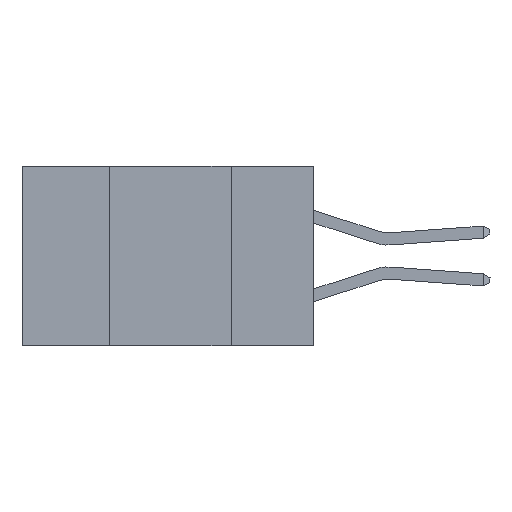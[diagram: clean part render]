
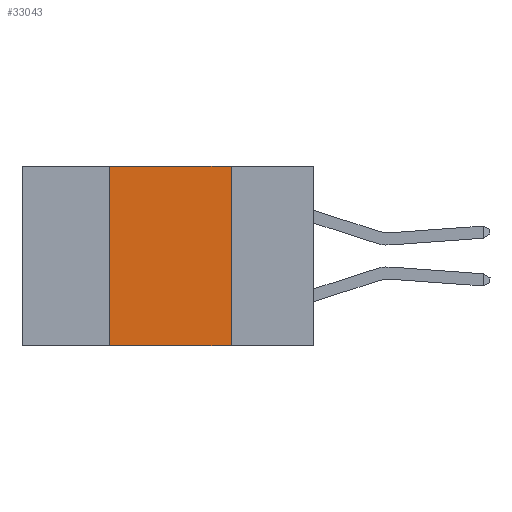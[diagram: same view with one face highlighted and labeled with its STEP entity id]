
A CAD part, left-side view. The second image highlights one B-rep face of the part: STEP entity #33043.
In plain terms, the highlighted planar face has unit normal (-1, 0, 0).
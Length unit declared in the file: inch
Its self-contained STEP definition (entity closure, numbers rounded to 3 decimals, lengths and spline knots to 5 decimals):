
#213 = PLANE ( 'NONE',  #12985 ) ;
#1413 = EDGE_CURVE ( 'NONE', #13924, #30875, #5237, .T. ) ;
#2487 = VERTEX_POINT ( 'NONE', #26704 ) ;
#2660 = CARTESIAN_POINT ( 'NONE',  ( 0., 0.17, -0.37 ) ) ;
#3637 = DIRECTION ( 'NONE',  ( 0., 0., -1. ) ) ;
#5237 = LINE ( 'NONE', #24204, #24035 ) ;
#6489 = DIRECTION ( 'NONE',  ( 0., -1., 0. ) ) ;
#6558 = CARTESIAN_POINT ( 'NONE',  ( 0., 0.6, 0. ) ) ;
#6837 = DIRECTION ( 'NONE',  ( 1., 0., 0. ) ) ;
#8653 = VECTOR ( 'NONE', #6489, 39.37008 ) ;
#9623 = ORIENTED_EDGE ( 'NONE', *, *, #11291, .F. ) ;
#9703 = VECTOR ( 'NONE', #27496, 39.37008 ) ;
#10065 = CARTESIAN_POINT ( 'NONE',  ( 0., 0.6, 0. ) ) ;
#11291 = EDGE_CURVE ( 'NONE', #2487, #30092, #21121, .T. ) ;
#12985 = AXIS2_PLACEMENT_3D ( 'NONE', #6558, #6837, #3637 ) ;
#13924 = VERTEX_POINT ( 'NONE', #15099 ) ;
#15099 = CARTESIAN_POINT ( 'NONE',  ( 0., 0.42, -0.37 ) ) ;
#15466 = DIRECTION ( 'NONE',  ( 0., -1., 0. ) ) ;
#18282 = ORIENTED_EDGE ( 'NONE', *, *, #26623, .T. ) ;
#20705 = LINE ( 'NONE', #34495, #27587 ) ;
#21121 = LINE ( 'NONE', #33683, #9703 ) ;
#22543 = ORIENTED_EDGE ( 'NONE', *, *, #38991, .F. ) ;
#24035 = VECTOR ( 'NONE', #30801, 39.37008 ) ;
#24204 = CARTESIAN_POINT ( 'NONE',  ( 0., 0.42, 0. ) ) ;
#25745 = ORIENTED_EDGE ( 'NONE', *, *, #1413, .F. ) ;
#26218 = EDGE_LOOP ( 'NONE', ( #9623, #22543, #25745, #18282 ) ) ;
#26623 = EDGE_CURVE ( 'NONE', #13924, #30092, #20705, .T. ) ;
#26704 = CARTESIAN_POINT ( 'NONE',  ( 0., 0.17, 0. ) ) ;
#27496 = DIRECTION ( 'NONE',  ( 0., 0., -1. ) ) ;
#27587 = VECTOR ( 'NONE', #15466, 39.37008 ) ;
#27610 = CARTESIAN_POINT ( 'NONE',  ( 0., 0.42, 0. ) ) ;
#29982 = LINE ( 'NONE', #10065, #8653 ) ;
#30092 = VERTEX_POINT ( 'NONE', #2660 ) ;
#30801 = DIRECTION ( 'NONE',  ( 0., 0., 1. ) ) ;
#30875 = VERTEX_POINT ( 'NONE', #27610 ) ;
#33043 = ADVANCED_FACE ( 'NONE', ( #33367 ), #213, .F. ) ;
#33367 = FACE_OUTER_BOUND ( 'NONE', #26218, .T. ) ;
#33683 = CARTESIAN_POINT ( 'NONE',  ( 0., 0.17, 0. ) ) ;
#34495 = CARTESIAN_POINT ( 'NONE',  ( 0., 0.6, -0.37 ) ) ;
#38991 = EDGE_CURVE ( 'NONE', #30875, #2487, #29982, .T. ) ;
